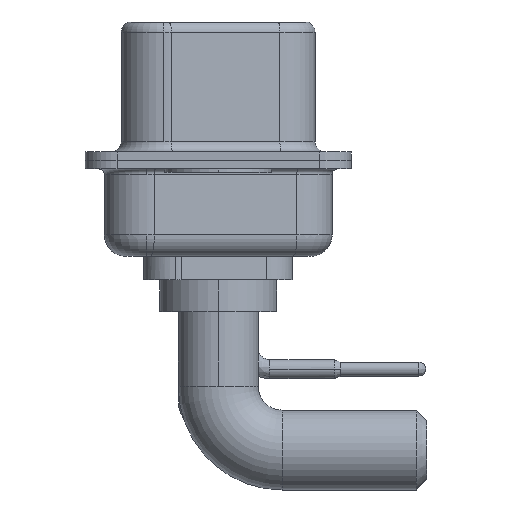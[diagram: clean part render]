
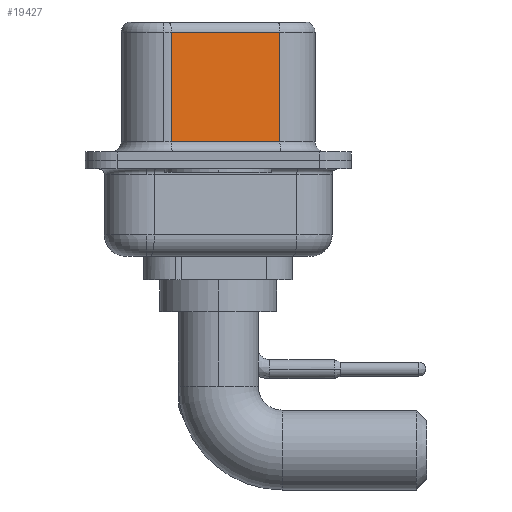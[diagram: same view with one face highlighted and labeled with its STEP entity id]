
A CAD part, left-side view. The second image highlights one B-rep face of the part: STEP entity #19427.
In plain terms, the highlighted planar face has unit normal (-0.985, -0.174, 0).
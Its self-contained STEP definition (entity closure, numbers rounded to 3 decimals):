
#710 = VECTOR ( 'NONE', #7904, 1000. ) ;
#1630 = CARTESIAN_POINT ( 'NONE',  ( 4.58, -2.897, 0.9 ) ) ;
#1638 = PLANE ( 'NONE',  #8156 ) ;
#1661 = LINE ( 'NONE', #4666, #710 ) ;
#1875 = EDGE_LOOP ( 'NONE', ( #17778, #13647, #8319, #14106 ) ) ;
#1931 = CARTESIAN_POINT ( 'NONE',  ( 4.58, -2.897, 0.9 ) ) ;
#3964 = VERTEX_POINT ( 'NONE', #6014 ) ;
#4150 = VECTOR ( 'NONE', #16463, 1000. ) ;
#4242 = EDGE_CURVE ( 'NONE', #9465, #9187, #10616, .T. ) ;
#4537 = LINE ( 'NONE', #1630, #8494 ) ;
#4666 = CARTESIAN_POINT ( 'NONE',  ( 4.58, -2.897, 6.02 ) ) ;
#5964 = VECTOR ( 'NONE', #19826, 1000. ) ;
#6014 = CARTESIAN_POINT ( 'NONE',  ( 3.68, 2.203, 0.9 ) ) ;
#7904 = DIRECTION ( 'NONE',  ( -0.174, 0.985, 0. ) ) ;
#8156 = AXIS2_PLACEMENT_3D ( 'NONE', #20643, #14179, #20438 ) ;
#8319 = ORIENTED_EDGE ( 'NONE', *, *, #19556, .T. ) ;
#8494 = VECTOR ( 'NONE', #15740, 1000. ) ;
#8914 = CARTESIAN_POINT ( 'NONE',  ( 4.58, -2.897, 6.02 ) ) ;
#9187 = VERTEX_POINT ( 'NONE', #1931 ) ;
#9452 = CARTESIAN_POINT ( 'NONE',  ( 3.68, 2.203, 6.02 ) ) ;
#9465 = VERTEX_POINT ( 'NONE', #8914 ) ;
#10616 = LINE ( 'NONE', #11978, #5964 ) ;
#11978 = CARTESIAN_POINT ( 'NONE',  ( 4.58, -2.897, 6.52 ) ) ;
#12402 = FACE_OUTER_BOUND ( 'NONE', #1875, .T. ) ;
#13265 = VERTEX_POINT ( 'NONE', #9452 ) ;
#13647 = ORIENTED_EDGE ( 'NONE', *, *, #14811, .T. ) ;
#14106 = ORIENTED_EDGE ( 'NONE', *, *, #18095, .T. ) ;
#14179 = DIRECTION ( 'NONE',  ( 0.985, 0.174, 0. ) ) ;
#14811 = EDGE_CURVE ( 'NONE', #9465, #13265, #1661, .T. ) ;
#15740 = DIRECTION ( 'NONE',  ( 0.174, -0.985, 0. ) ) ;
#16463 = DIRECTION ( 'NONE',  ( 0., 0., -1. ) ) ;
#17778 = ORIENTED_EDGE ( 'NONE', *, *, #4242, .F. ) ;
#18095 = EDGE_CURVE ( 'NONE', #3964, #9187, #4537, .T. ) ;
#19427 = ADVANCED_FACE ( 'NONE', ( #12402 ), #1638, .F. ) ;
#19501 = CARTESIAN_POINT ( 'NONE',  ( 3.68, 2.203, 6.52 ) ) ;
#19556 = EDGE_CURVE ( 'NONE', #13265, #3964, #19702, .T. ) ;
#19702 = LINE ( 'NONE', #19501, #4150 ) ;
#19826 = DIRECTION ( 'NONE',  ( 0., 0., -1. ) ) ;
#20438 = DIRECTION ( 'NONE',  ( -0.174, 0.985, 0. ) ) ;
#20643 = CARTESIAN_POINT ( 'NONE',  ( 4.58, -2.897, 6.52 ) ) ;
